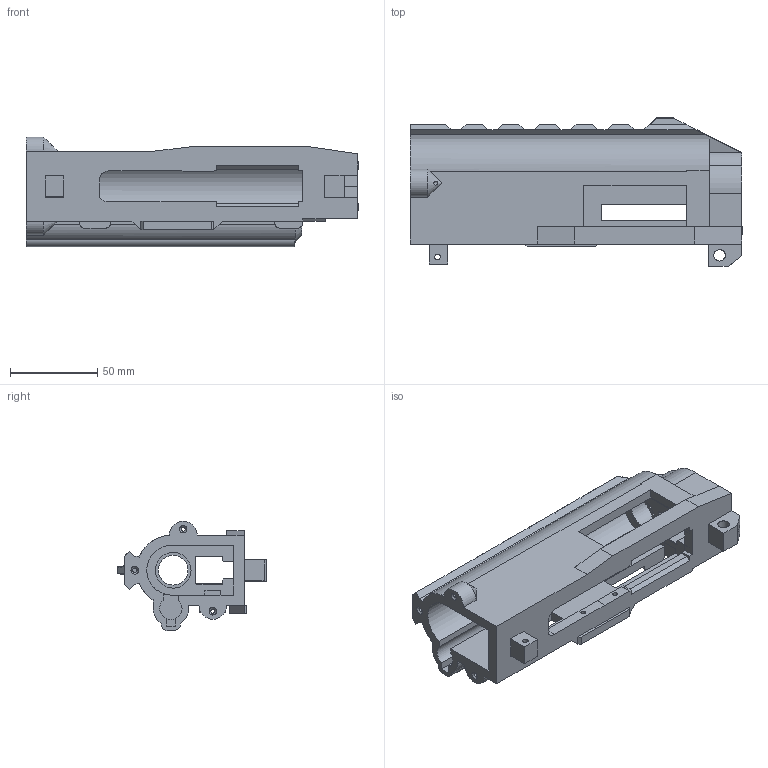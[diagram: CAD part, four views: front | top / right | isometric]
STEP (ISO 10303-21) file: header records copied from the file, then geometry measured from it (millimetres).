
FILE_DESCRIPTION(('FreeCAD Model'),'2;1');
FILE_NAME( 'latest hillbilly upper.step', '2020-08-12T17:29:07',('Author'),(''), 'Open CASCADE STEP processor 6.8','FreeCAD','Unknown');
FILE_SCHEMA(('AUTOMOTIVE_DESIGN_CC2 { 1 2 10303 214 -1 1 5 4 }'));
Length unit declared in the file: millimetre
Products named in the file (1): Pocket004
Bounding box: 190.38 x 85.37 x 62.82 mm (x, y, z)
Volume: 218046.4 mm3; surface area: 80049.3 mm2
Topology: 1 solids, 2 shells, 339 faces, 947 edges, 618 vertices
Faces by surface type: plane 271, cylinder 56, cone 10, bspline 2
Full cylindrical faces by diameter (mm): 2 x1, 2.2 x1, 2.4 x5, 2.5 x1, 2.6 x2, 3.175 x1, 6.6 x1, 17 x1, 20.49 x1
Entity records: 35885 total; most frequent: CARTESIAN_POINT 17590, DIRECTION 3138, LINE 2239, VECTOR 2239, ORIENTED_EDGE 1892, PCURVE 1892, DEFINITIONAL_REPRESENTATION 1892, EDGE_CURVE 946
